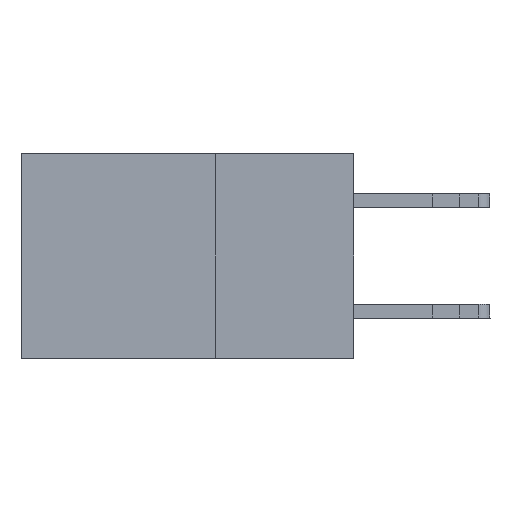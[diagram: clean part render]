
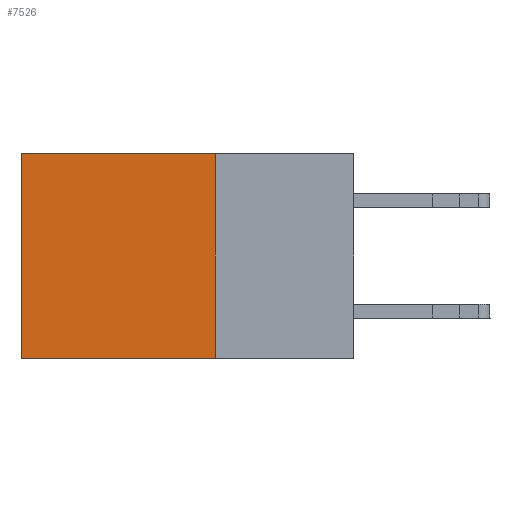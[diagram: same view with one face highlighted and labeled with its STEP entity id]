
A CAD part, left-side view. The second image highlights one B-rep face of the part: STEP entity #7526.
In plain terms, the highlighted planar face has unit normal (-1, 0, 0).
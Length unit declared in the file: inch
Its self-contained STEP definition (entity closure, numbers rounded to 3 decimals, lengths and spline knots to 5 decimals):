
#195 = CARTESIAN_POINT ( 'NONE',  ( 0.2875, 0.25, 0. ) ) ;
#1009 = EDGE_CURVE ( 'NONE', #18633, #15593, #20560, .T. ) ;
#2540 = DIRECTION ( 'NONE',  ( 0., 0., -1. ) ) ;
#3087 = CARTESIAN_POINT ( 'NONE',  ( 0.2875, 0.25, 0. ) ) ;
#3163 = VECTOR ( 'NONE', #10582, 39.37008 ) ;
#3984 = CARTESIAN_POINT ( 'NONE',  ( 0.2875, 0.6, 0. ) ) ;
#5087 = DIRECTION ( 'NONE',  ( 0., 0., -1. ) ) ;
#5126 = ORIENTED_EDGE ( 'NONE', *, *, #22630, .T. ) ;
#7526 = ADVANCED_FACE ( 'NONE', ( #9856 ), #10037, .F. ) ;
#7692 = LINE ( 'NONE', #3087, #22030 ) ;
#7795 = VERTEX_POINT ( 'NONE', #9812 ) ;
#9352 = VECTOR ( 'NONE', #23401, 39.37008 ) ;
#9758 = DIRECTION ( 'NONE',  ( 0., 0., -1. ) ) ;
#9812 = CARTESIAN_POINT ( 'NONE',  ( 0.2875, 0.25, 0. ) ) ;
#9856 = FACE_OUTER_BOUND ( 'NONE', #21657, .T. ) ;
#10037 = PLANE ( 'NONE',  #20352 ) ;
#10316 = ORIENTED_EDGE ( 'NONE', *, *, #10826, .F. ) ;
#10582 = DIRECTION ( 'NONE',  ( 0., 1., 0. ) ) ;
#10826 = EDGE_CURVE ( 'NONE', #7795, #18633, #7692, .T. ) ;
#12451 = CARTESIAN_POINT ( 'NONE',  ( 0.2875, 0.6, -0.37 ) ) ;
#12569 = CARTESIAN_POINT ( 'NONE',  ( 0.2875, 0.25, 0. ) ) ;
#15025 = VERTEX_POINT ( 'NONE', #3984 ) ;
#15593 = VERTEX_POINT ( 'NONE', #12451 ) ;
#16233 = ORIENTED_EDGE ( 'NONE', *, *, #1009, .F. ) ;
#16744 = EDGE_CURVE ( 'NONE', #7795, #15025, #18175, .T. ) ;
#17649 = CARTESIAN_POINT ( 'NONE',  ( 0.2875, 0.25, -0.37 ) ) ;
#18175 = LINE ( 'NONE', #12569, #3163 ) ;
#18237 = VECTOR ( 'NONE', #9758, 39.37008 ) ;
#18633 = VERTEX_POINT ( 'NONE', #23281 ) ;
#20348 = CARTESIAN_POINT ( 'NONE',  ( 0.2875, 0.6, 0. ) ) ;
#20352 = AXIS2_PLACEMENT_3D ( 'NONE', #195, #24568, #2540 ) ;
#20560 = LINE ( 'NONE', #17649, #9352 ) ;
#21657 = EDGE_LOOP ( 'NONE', ( #5126, #16233, #10316, #23344 ) ) ;
#22030 = VECTOR ( 'NONE', #5087, 39.37008 ) ;
#22630 = EDGE_CURVE ( 'NONE', #15025, #15593, #24692, .T. ) ;
#23281 = CARTESIAN_POINT ( 'NONE',  ( 0.2875, 0.25, -0.37 ) ) ;
#23344 = ORIENTED_EDGE ( 'NONE', *, *, #16744, .T. ) ;
#23401 = DIRECTION ( 'NONE',  ( 0., 1., 0. ) ) ;
#24568 = DIRECTION ( 'NONE',  ( 1., 0., 0. ) ) ;
#24692 = LINE ( 'NONE', #20348, #18237 ) ;
